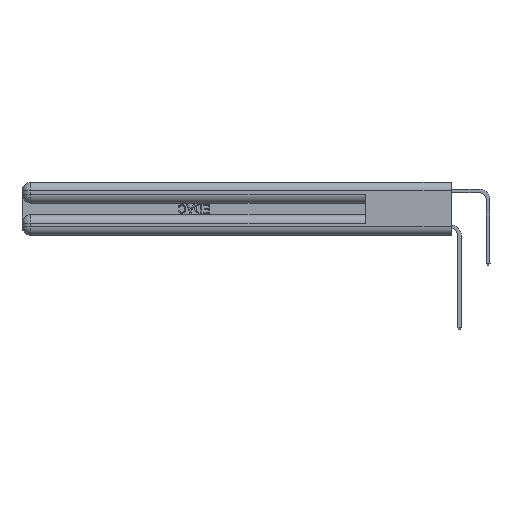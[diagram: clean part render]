
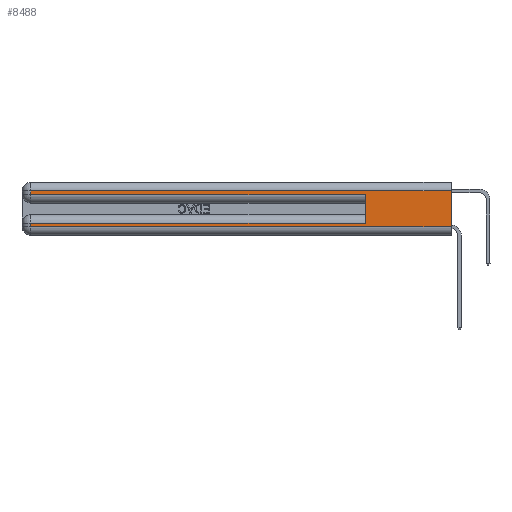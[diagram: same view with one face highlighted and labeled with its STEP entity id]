
A CAD part, left-side view. The second image highlights one B-rep face of the part: STEP entity #8488.
In plain terms, the highlighted planar face has unit normal (-1, 0, 0).
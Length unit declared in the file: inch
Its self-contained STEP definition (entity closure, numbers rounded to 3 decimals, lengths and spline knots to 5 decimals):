
#255 = VERTEX_POINT ( 'NONE', #19216 ) ;
#398 = VERTEX_POINT ( 'NONE', #987 ) ;
#418 = VECTOR ( 'NONE', #8846, 39.37008 ) ;
#609 = CARTESIAN_POINT ( 'NONE',  ( 0., 2.94, 0.37 ) ) ;
#987 = CARTESIAN_POINT ( 'NONE',  ( 0., 0., 0.31 ) ) ;
#1437 = VECTOR ( 'NONE', #2558, 39.37008 ) ;
#1756 = DIRECTION ( 'NONE',  ( 0., -1., 0. ) ) ;
#2117 = VERTEX_POINT ( 'NONE', #18510 ) ;
#2558 = DIRECTION ( 'NONE',  ( 0., 1., 0. ) ) ;
#2981 = CARTESIAN_POINT ( 'NONE',  ( 0., 0., 0.31 ) ) ;
#3688 = CARTESIAN_POINT ( 'NONE',  ( 0., 0.6, 0.145 ) ) ;
#3702 = LINE ( 'NONE', #13914, #30662 ) ;
#5791 = DIRECTION ( 'NONE',  ( 0., 1., 0. ) ) ;
#6666 = ORIENTED_EDGE ( 'NONE', *, *, #28576, .T. ) ;
#6863 = VERTEX_POINT ( 'NONE', #13680 ) ;
#7163 = DIRECTION ( 'NONE',  ( 0., -1., 0. ) ) ;
#8267 = CARTESIAN_POINT ( 'NONE',  ( 0., 2.94, 0.085 ) ) ;
#8488 = ADVANCED_FACE ( 'NONE', ( #11070 ), #15619, .F. ) ;
#8846 = DIRECTION ( 'NONE',  ( 0., 0., 1. ) ) ;
#9176 = EDGE_LOOP ( 'NONE', ( #30610, #23036, #6666, #29739, #29832, #24132, #13291, #29496 ) ) ;
#9451 = LINE ( 'NONE', #17808, #14126 ) ;
#11070 = FACE_OUTER_BOUND ( 'NONE', #9176, .T. ) ;
#11735 = EDGE_CURVE ( 'NONE', #21862, #25967, #16117, .T. ) ;
#11849 = AXIS2_PLACEMENT_3D ( 'NONE', #17914, #20552, #25137 ) ;
#12996 = EDGE_CURVE ( 'NONE', #398, #6863, #9451, .T. ) ;
#13154 = EDGE_CURVE ( 'NONE', #21862, #30995, #18815, .T. ) ;
#13291 = ORIENTED_EDGE ( 'NONE', *, *, #25997, .T. ) ;
#13438 = VECTOR ( 'NONE', #13454, 39.37008 ) ;
#13454 = DIRECTION ( 'NONE',  ( 0., 0., -1. ) ) ;
#13680 = CARTESIAN_POINT ( 'NONE',  ( 0., 0., 0.06 ) ) ;
#13914 = CARTESIAN_POINT ( 'NONE',  ( 0., 0., 0.06 ) ) ;
#14126 = VECTOR ( 'NONE', #28923, 39.37008 ) ;
#14769 = VECTOR ( 'NONE', #15825, 39.37008 ) ;
#15541 = LINE ( 'NONE', #2981, #1437 ) ;
#15619 = PLANE ( 'NONE',  #11849 ) ;
#15633 = VERTEX_POINT ( 'NONE', #31275 ) ;
#15825 = DIRECTION ( 'NONE',  ( 0., 0., -1. ) ) ;
#16117 = LINE ( 'NONE', #23319, #31309 ) ;
#16934 = EDGE_CURVE ( 'NONE', #255, #6863, #3702, .T. ) ;
#17648 = CARTESIAN_POINT ( 'NONE',  ( 0., 0., 0.285 ) ) ;
#17808 = CARTESIAN_POINT ( 'NONE',  ( 0., 0., 0.37 ) ) ;
#17914 = CARTESIAN_POINT ( 'NONE',  ( 0., 0., 0.37 ) ) ;
#18510 = CARTESIAN_POINT ( 'NONE',  ( 0., 2.94, 0.31 ) ) ;
#18815 = LINE ( 'NONE', #3688, #418 ) ;
#19216 = CARTESIAN_POINT ( 'NONE',  ( 0., 2.94, 0.06 ) ) ;
#20552 = DIRECTION ( 'NONE',  ( 1., 0., 0. ) ) ;
#21074 = CARTESIAN_POINT ( 'NONE',  ( 0., 0.6, 0.085 ) ) ;
#21862 = VERTEX_POINT ( 'NONE', #21074 ) ;
#22771 = CARTESIAN_POINT ( 'NONE',  ( 0., 0.6, 0.285 ) ) ;
#23036 = ORIENTED_EDGE ( 'NONE', *, *, #26508, .T. ) ;
#23319 = CARTESIAN_POINT ( 'NONE',  ( 0., 0., 0.085 ) ) ;
#24132 = ORIENTED_EDGE ( 'NONE', *, *, #11735, .T. ) ;
#24653 = EDGE_CURVE ( 'NONE', #15633, #30995, #29664, .T. ) ;
#25137 = DIRECTION ( 'NONE',  ( 0., 0., -1. ) ) ;
#25967 = VERTEX_POINT ( 'NONE', #8267 ) ;
#25997 = EDGE_CURVE ( 'NONE', #25967, #255, #28075, .T. ) ;
#26140 = CARTESIAN_POINT ( 'NONE',  ( 0., 2.94, 0.37 ) ) ;
#26508 = EDGE_CURVE ( 'NONE', #398, #2117, #15541, .T. ) ;
#28075 = LINE ( 'NONE', #609, #14769 ) ;
#28576 = EDGE_CURVE ( 'NONE', #2117, #15633, #31767, .T. ) ;
#28923 = DIRECTION ( 'NONE',  ( 0., 0., -1. ) ) ;
#29496 = ORIENTED_EDGE ( 'NONE', *, *, #16934, .T. ) ;
#29664 = LINE ( 'NONE', #17648, #30434 ) ;
#29739 = ORIENTED_EDGE ( 'NONE', *, *, #24653, .T. ) ;
#29832 = ORIENTED_EDGE ( 'NONE', *, *, #13154, .F. ) ;
#30434 = VECTOR ( 'NONE', #7163, 39.37008 ) ;
#30610 = ORIENTED_EDGE ( 'NONE', *, *, #12996, .F. ) ;
#30662 = VECTOR ( 'NONE', #1756, 39.37008 ) ;
#30995 = VERTEX_POINT ( 'NONE', #22771 ) ;
#31275 = CARTESIAN_POINT ( 'NONE',  ( 0., 2.94, 0.285 ) ) ;
#31309 = VECTOR ( 'NONE', #5791, 39.37008 ) ;
#31767 = LINE ( 'NONE', #26140, #13438 ) ;
